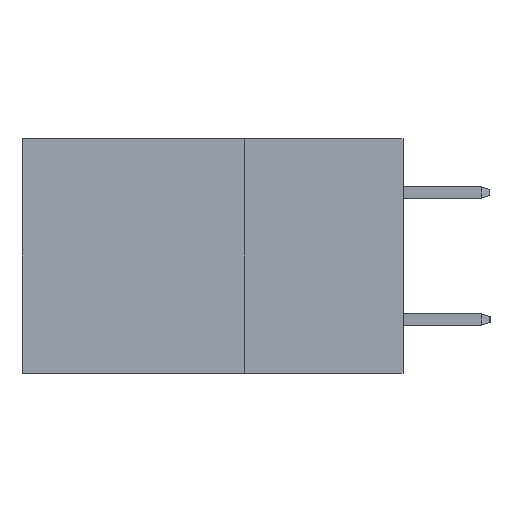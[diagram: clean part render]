
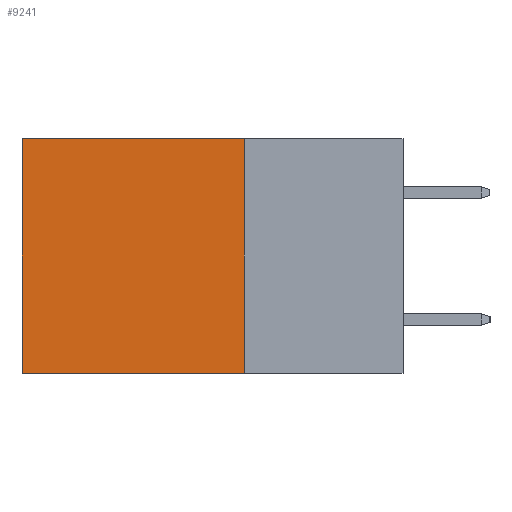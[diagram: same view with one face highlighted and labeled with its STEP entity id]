
A CAD part, left-side view. The second image highlights one B-rep face of the part: STEP entity #9241.
In plain terms, the highlighted planar face has unit normal (-1, 0, 0).
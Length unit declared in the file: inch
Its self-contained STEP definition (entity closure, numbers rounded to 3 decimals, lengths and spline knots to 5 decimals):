
#720 = PLANE ( 'NONE',  #12018 ) ;
#920 = DIRECTION ( 'NONE',  ( 1., 0., 0. ) ) ;
#1246 = DIRECTION ( 'NONE',  ( 0., 0., -1. ) ) ;
#1473 = CARTESIAN_POINT ( 'NONE',  ( 0.2875, 0.25, -0.37 ) ) ;
#1543 = CARTESIAN_POINT ( 'NONE',  ( 0.2875, 0.25, 0. ) ) ;
#1966 = EDGE_CURVE ( 'NONE', #8405, #9551, #9147, .T. ) ;
#2069 = LINE ( 'NONE', #6449, #2455 ) ;
#2455 = VECTOR ( 'NONE', #3595, 39.37008 ) ;
#2724 = CARTESIAN_POINT ( 'NONE',  ( 0.2875, 0.25, 0. ) ) ;
#3086 = DIRECTION ( 'NONE',  ( 0., 1., 0. ) ) ;
#3595 = DIRECTION ( 'NONE',  ( 0., 0., -1. ) ) ;
#4054 = DIRECTION ( 'NONE',  ( 0., 1., 0. ) ) ;
#4837 = CARTESIAN_POINT ( 'NONE',  ( 0.2875, 0.6, -0.37 ) ) ;
#5354 = CARTESIAN_POINT ( 'NONE',  ( 0.2875, 0.25, -0.37 ) ) ;
#5483 = FACE_OUTER_BOUND ( 'NONE', #14640, .T. ) ;
#5555 = VECTOR ( 'NONE', #3086, 39.37008 ) ;
#6336 = ORIENTED_EDGE ( 'NONE', *, *, #10364, .F. ) ;
#6366 = CARTESIAN_POINT ( 'NONE',  ( 0.2875, 0.6, 0. ) ) ;
#6449 = CARTESIAN_POINT ( 'NONE',  ( 0.2875, 0.6, 0. ) ) ;
#7653 = VECTOR ( 'NONE', #1246, 39.37008 ) ;
#7864 = LINE ( 'NONE', #1473, #5555 ) ;
#8405 = VERTEX_POINT ( 'NONE', #16429 ) ;
#9147 = LINE ( 'NONE', #1543, #7653 ) ;
#9241 = ADVANCED_FACE ( 'NONE', ( #5483 ), #720, .F. ) ;
#9429 = EDGE_CURVE ( 'NONE', #8405, #16387, #10457, .T. ) ;
#9551 = VERTEX_POINT ( 'NONE', #5354 ) ;
#10364 = EDGE_CURVE ( 'NONE', #9551, #11234, #7864, .T. ) ;
#10457 = LINE ( 'NONE', #2724, #18869 ) ;
#11234 = VERTEX_POINT ( 'NONE', #4837 ) ;
#12018 = AXIS2_PLACEMENT_3D ( 'NONE', #17570, #920, #13012 ) ;
#13012 = DIRECTION ( 'NONE',  ( 0., 0., -1. ) ) ;
#13713 = ORIENTED_EDGE ( 'NONE', *, *, #9429, .T. ) ;
#14640 = EDGE_LOOP ( 'NONE', ( #17903, #6336, #18388, #13713 ) ) ;
#16387 = VERTEX_POINT ( 'NONE', #6366 ) ;
#16429 = CARTESIAN_POINT ( 'NONE',  ( 0.2875, 0.25, 0. ) ) ;
#16939 = EDGE_CURVE ( 'NONE', #16387, #11234, #2069, .T. ) ;
#17570 = CARTESIAN_POINT ( 'NONE',  ( 0.2875, 0.25, 0. ) ) ;
#17903 = ORIENTED_EDGE ( 'NONE', *, *, #16939, .T. ) ;
#18388 = ORIENTED_EDGE ( 'NONE', *, *, #1966, .F. ) ;
#18869 = VECTOR ( 'NONE', #4054, 39.37008 ) ;
